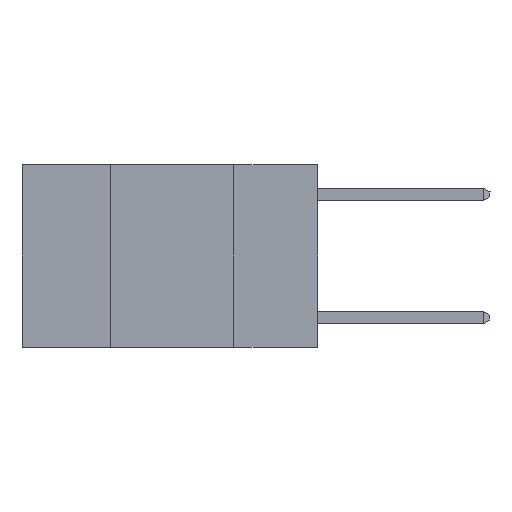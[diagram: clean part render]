
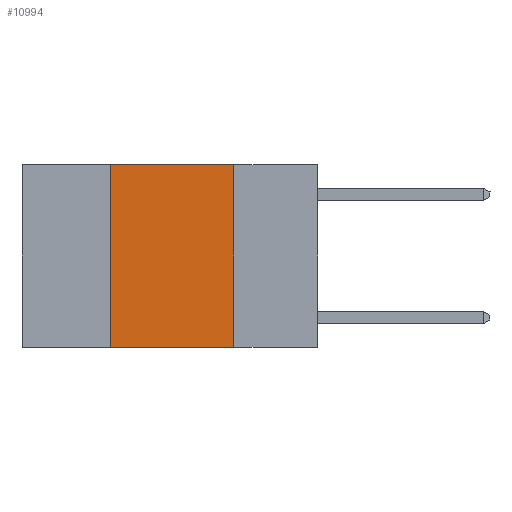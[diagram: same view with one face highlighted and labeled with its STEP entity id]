
A CAD part, left-side view. The second image highlights one B-rep face of the part: STEP entity #10994.
In plain terms, the highlighted planar face has unit normal (-1, 0, 0).
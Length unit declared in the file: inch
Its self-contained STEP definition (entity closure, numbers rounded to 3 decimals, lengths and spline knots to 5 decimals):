
#530 = LINE ( 'NONE', #2617, #3233 ) ;
#733 = DIRECTION ( 'NONE',  ( 0., 0., 1. ) ) ;
#747 = DIRECTION ( 'NONE',  ( 0., -1., 0. ) ) ;
#1588 = PLANE ( 'NONE',  #2586 ) ;
#2586 = AXIS2_PLACEMENT_3D ( 'NONE', #2732, #3877, #11071 ) ;
#2617 = CARTESIAN_POINT ( 'NONE',  ( 0., 0.17, 0. ) ) ;
#2732 = CARTESIAN_POINT ( 'NONE',  ( 0., 0.6, 0. ) ) ;
#2849 = EDGE_CURVE ( 'NONE', #3581, #6561, #6530, .T. ) ;
#2896 = ORIENTED_EDGE ( 'NONE', *, *, #2849, .F. ) ;
#3139 = VERTEX_POINT ( 'NONE', #12058 ) ;
#3233 = VECTOR ( 'NONE', #9898, 39.37008 ) ;
#3406 = LINE ( 'NONE', #7205, #5583 ) ;
#3581 = VERTEX_POINT ( 'NONE', #8450 ) ;
#3815 = VECTOR ( 'NONE', #4596, 39.37008 ) ;
#3877 = DIRECTION ( 'NONE',  ( 1., 0., 0. ) ) ;
#4596 = DIRECTION ( 'NONE',  ( 0., -1., 0. ) ) ;
#5167 = ORIENTED_EDGE ( 'NONE', *, *, #9919, .F. ) ;
#5583 = VECTOR ( 'NONE', #733, 39.37008 ) ;
#5760 = EDGE_LOOP ( 'NONE', ( #10082, #2896, #5167, #7532 ) ) ;
#5944 = CARTESIAN_POINT ( 'NONE',  ( 0., 0.17, -0.37 ) ) ;
#6530 = LINE ( 'NONE', #12653, #3815 ) ;
#6561 = VERTEX_POINT ( 'NONE', #6870 ) ;
#6870 = CARTESIAN_POINT ( 'NONE',  ( 0., 0.17, 0. ) ) ;
#7205 = CARTESIAN_POINT ( 'NONE',  ( 0., 0.42, 0. ) ) ;
#7532 = ORIENTED_EDGE ( 'NONE', *, *, #11219, .T. ) ;
#7897 = VECTOR ( 'NONE', #747, 39.37008 ) ;
#8251 = CARTESIAN_POINT ( 'NONE',  ( 0., 0.6, -0.37 ) ) ;
#8450 = CARTESIAN_POINT ( 'NONE',  ( 0., 0.42, 0. ) ) ;
#9528 = VERTEX_POINT ( 'NONE', #5944 ) ;
#9724 = EDGE_CURVE ( 'NONE', #6561, #9528, #530, .T. ) ;
#9898 = DIRECTION ( 'NONE',  ( 0., 0., -1. ) ) ;
#9919 = EDGE_CURVE ( 'NONE', #3139, #3581, #3406, .T. ) ;
#10082 = ORIENTED_EDGE ( 'NONE', *, *, #9724, .F. ) ;
#10136 = FACE_OUTER_BOUND ( 'NONE', #5760, .T. ) ;
#10994 = ADVANCED_FACE ( 'NONE', ( #10136 ), #1588, .F. ) ;
#11071 = DIRECTION ( 'NONE',  ( 0., 0., -1. ) ) ;
#11219 = EDGE_CURVE ( 'NONE', #3139, #9528, #12978, .T. ) ;
#12058 = CARTESIAN_POINT ( 'NONE',  ( 0., 0.42, -0.37 ) ) ;
#12653 = CARTESIAN_POINT ( 'NONE',  ( 0., 0.6, 0. ) ) ;
#12978 = LINE ( 'NONE', #8251, #7897 ) ;
